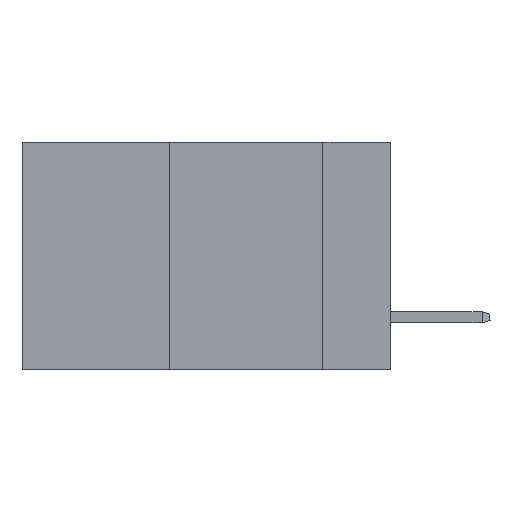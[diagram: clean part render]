
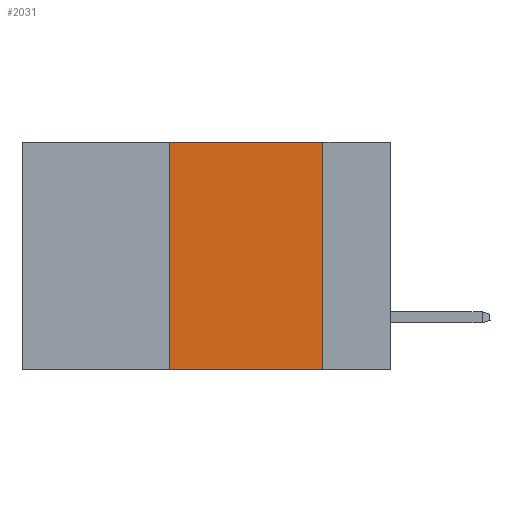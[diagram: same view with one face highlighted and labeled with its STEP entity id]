
A CAD part, left-side view. The second image highlights one B-rep face of the part: STEP entity #2031.
In plain terms, the highlighted planar face has unit normal (-1, 0, 0).
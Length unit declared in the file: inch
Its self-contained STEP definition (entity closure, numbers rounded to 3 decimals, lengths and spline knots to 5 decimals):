
#347 = VERTEX_POINT ( 'NONE', #6798 ) ;
#1127 = VECTOR ( 'NONE', #13401, 39.37008 ) ;
#1544 = DIRECTION ( 'NONE',  ( 1., 0., 0. ) ) ;
#1773 = CARTESIAN_POINT ( 'NONE',  ( 0., 0.6, 0. ) ) ;
#2031 = ADVANCED_FACE ( 'NONE', ( #8513 ), #6821, .F. ) ;
#4609 = ORIENTED_EDGE ( 'NONE', *, *, #16708, .F. ) ;
#5237 = LINE ( 'NONE', #14066, #17540 ) ;
#5701 = VECTOR ( 'NONE', #17607, 39.37008 ) ;
#5712 = VERTEX_POINT ( 'NONE', #12894 ) ;
#6392 = CARTESIAN_POINT ( 'NONE',  ( 0., 0.11, 0. ) ) ;
#6798 = CARTESIAN_POINT ( 'NONE',  ( 0., 0.11, 0. ) ) ;
#6821 = PLANE ( 'NONE',  #18579 ) ;
#7698 = EDGE_LOOP ( 'NONE', ( #13730, #4609, #8700, #18856 ) ) ;
#8513 = FACE_OUTER_BOUND ( 'NONE', #7698, .T. ) ;
#8694 = EDGE_CURVE ( 'NONE', #5712, #8855, #13665, .T. ) ;
#8700 = ORIENTED_EDGE ( 'NONE', *, *, #20281, .F. ) ;
#8855 = VERTEX_POINT ( 'NONE', #19967 ) ;
#11023 = CARTESIAN_POINT ( 'NONE',  ( 0., 0.36, 0. ) ) ;
#11835 = CARTESIAN_POINT ( 'NONE',  ( 0., 0.6, -0.37 ) ) ;
#12894 = CARTESIAN_POINT ( 'NONE',  ( 0., 0.36, -0.37 ) ) ;
#13401 = DIRECTION ( 'NONE',  ( 0., -1., 0. ) ) ;
#13665 = LINE ( 'NONE', #11835, #1127 ) ;
#13730 = ORIENTED_EDGE ( 'NONE', *, *, #17482, .F. ) ;
#14066 = CARTESIAN_POINT ( 'NONE',  ( 0., 0.6, 0. ) ) ;
#14310 = LINE ( 'NONE', #6392, #5701 ) ;
#15706 = DIRECTION ( 'NONE',  ( 0., -1., 0. ) ) ;
#16588 = DIRECTION ( 'NONE',  ( 0., 0., -1. ) ) ;
#16635 = VERTEX_POINT ( 'NONE', #19998 ) ;
#16708 = EDGE_CURVE ( 'NONE', #16635, #347, #5237, .T. ) ;
#17482 = EDGE_CURVE ( 'NONE', #347, #8855, #14310, .T. ) ;
#17540 = VECTOR ( 'NONE', #15706, 39.37008 ) ;
#17607 = DIRECTION ( 'NONE',  ( 0., 0., -1. ) ) ;
#18310 = VECTOR ( 'NONE', #18850, 39.37008 ) ;
#18579 = AXIS2_PLACEMENT_3D ( 'NONE', #1773, #1544, #16588 ) ;
#18850 = DIRECTION ( 'NONE',  ( 0., 0., 1. ) ) ;
#18856 = ORIENTED_EDGE ( 'NONE', *, *, #8694, .T. ) ;
#19233 = LINE ( 'NONE', #11023, #18310 ) ;
#19967 = CARTESIAN_POINT ( 'NONE',  ( 0., 0.11, -0.37 ) ) ;
#19998 = CARTESIAN_POINT ( 'NONE',  ( 0., 0.36, 0. ) ) ;
#20281 = EDGE_CURVE ( 'NONE', #5712, #16635, #19233, .T. ) ;
